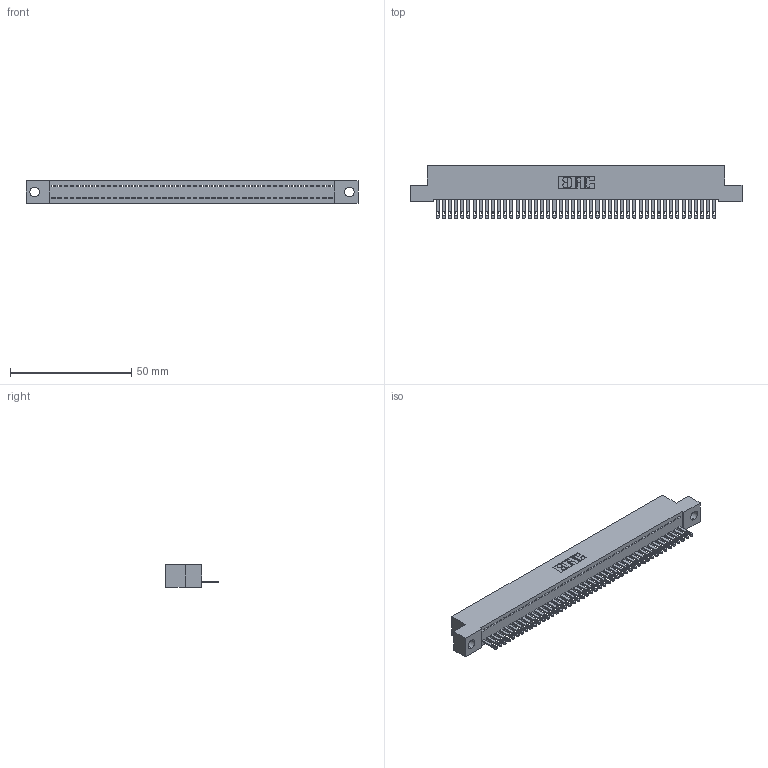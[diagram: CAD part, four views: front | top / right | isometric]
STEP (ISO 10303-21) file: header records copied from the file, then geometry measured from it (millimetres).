
FILE_DESCRIPTION (( 'STEP AP203' ), '1' );
FILE_NAME ('342-046-500-104.STEP', '2019-10-02T20:08:27', ( '' ), ( '' ), 'SwSTEP 2.0', 'SolidWorks 2016', '' );
FILE_SCHEMA (( 'CONFIG_CONTROL_DESIGN' ));
Length unit declared in the file: inch
Products named in the file (3): 342 Part_.156 TH; 345-292-001_345-293-100; 342-046-500-104
Assembly tree (47 placements, depth 2):
  342-046-500-104
    342 Part_.156 TH
    345-292-001_345-293-100  x46
Bounding box: 137.16 x 21.85 x 9.4 mm (x, y, z)
Volume: 11982.4 mm3; surface area: 17579.6 mm2
Topology: 47 solids, 47 shells, 2594 faces, 8027 edges, 5350 vertices
Faces by surface type: plane 1722, cylinder 872
Entity records: 27405 total; most frequent: CARTESIAN_POINT 4732, ORIENTED_EDGE 4714, DIRECTION 3985, EDGE_CURVE 2357, LINE 2225, VECTOR 2225, VERTEX_POINT 1570, AXIS2_PLACEMENT_3D 880
